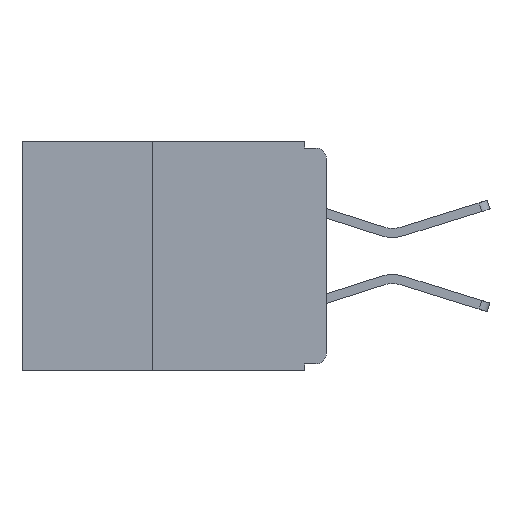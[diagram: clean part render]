
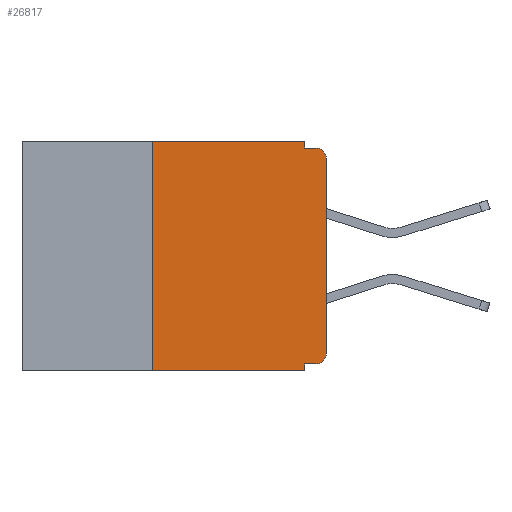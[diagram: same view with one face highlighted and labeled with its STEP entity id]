
A CAD part, left-side view. The second image highlights one B-rep face of the part: STEP entity #26817.
In plain terms, the highlighted planar face has unit normal (-1, 0, 0).
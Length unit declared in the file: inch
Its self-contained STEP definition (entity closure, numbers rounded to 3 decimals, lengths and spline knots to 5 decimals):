
#557 = DIRECTION ( 'NONE',  ( 0., 0., -1. ) ) ;
#1040 = CARTESIAN_POINT ( 'NONE',  ( 0., 0.25, -0.33 ) ) ;
#1101 = ORIENTED_EDGE ( 'NONE', *, *, #28838, .T. ) ;
#1144 = VECTOR ( 'NONE', #1265, 39.37008 ) ;
#1265 = DIRECTION ( 'NONE',  ( 0., -1., 0. ) ) ;
#1448 = CARTESIAN_POINT ( 'NONE',  ( 0., 0.437, 0. ) ) ;
#2435 = AXIS2_PLACEMENT_3D ( 'NONE', #10925, #27339, #13298 ) ;
#3317 = CARTESIAN_POINT ( 'NONE',  ( 0., 0.031, -0.33 ) ) ;
#3629 = AXIS2_PLACEMENT_3D ( 'NONE', #13656, #29959, #16044 ) ;
#4283 = FACE_OUTER_BOUND ( 'NONE', #9705, .T. ) ;
#4309 = CIRCLE ( 'NONE', #2435, 0.015 ) ;
#4609 = LINE ( 'NONE', #1040, #6136 ) ;
#4827 = CARTESIAN_POINT ( 'NONE',  ( 0., 0.437, -0.33 ) ) ;
#5340 = ORIENTED_EDGE ( 'NONE', *, *, #13169, .F. ) ;
#5691 = ORIENTED_EDGE ( 'NONE', *, *, #6755, .T. ) ;
#5757 = DIRECTION ( 'NONE',  ( 0., 0., -1. ) ) ;
#5878 = VERTEX_POINT ( 'NONE', #7886 ) ;
#5904 = DIRECTION ( 'NONE',  ( 0., 0., 1. ) ) ;
#6136 = VECTOR ( 'NONE', #5904, 39.37008 ) ;
#6251 = VECTOR ( 'NONE', #20528, 39.37008 ) ;
#6602 = VECTOR ( 'NONE', #28441, 39.37008 ) ;
#6671 = VERTEX_POINT ( 'NONE', #20366 ) ;
#6755 = EDGE_CURVE ( 'NONE', #5878, #24938, #7112, .T. ) ;
#7112 = CIRCLE ( 'NONE', #3629, 0.015 ) ;
#7171 = CARTESIAN_POINT ( 'NONE',  ( 0., 0.031, -0.33 ) ) ;
#7465 = CARTESIAN_POINT ( 'NONE',  ( 0., 0.25, -0.33 ) ) ;
#7669 = CARTESIAN_POINT ( 'NONE',  ( 0., 0., -0.305 ) ) ;
#7886 = CARTESIAN_POINT ( 'NONE',  ( 0., 0.015, -0.32 ) ) ;
#7937 = VECTOR ( 'NONE', #30121, 39.37008 ) ;
#8314 = CARTESIAN_POINT ( 'NONE',  ( 0., 0., -0.025 ) ) ;
#8569 = CARTESIAN_POINT ( 'NONE',  ( 0., 0., -0.01 ) ) ;
#9251 = ORIENTED_EDGE ( 'NONE', *, *, #11763, .F. ) ;
#9355 = LINE ( 'NONE', #3317, #21174 ) ;
#9705 = EDGE_LOOP ( 'NONE', ( #1101, #9840, #13151, #24404, #18712, #21427, #24216, #9251, #5340, #5691 ) ) ;
#9840 = ORIENTED_EDGE ( 'NONE', *, *, #9993, .T. ) ;
#9993 = EDGE_CURVE ( 'NONE', #22914, #6671, #4309, .T. ) ;
#10048 = CARTESIAN_POINT ( 'NONE',  ( 0., 0.031, -0.32 ) ) ;
#10231 = VECTOR ( 'NONE', #23945, 39.37008 ) ;
#10925 = CARTESIAN_POINT ( 'NONE',  ( 0., 0.015, -0.025 ) ) ;
#10972 = LINE ( 'NONE', #19273, #10231 ) ;
#11763 = EDGE_CURVE ( 'NONE', #19032, #14661, #9355, .T. ) ;
#12555 = PLANE ( 'NONE',  #16244 ) ;
#12974 = LINE ( 'NONE', #4827, #6602 ) ;
#13127 = EDGE_CURVE ( 'NONE', #30476, #18614, #13366, .T. ) ;
#13151 = ORIENTED_EDGE ( 'NONE', *, *, #21045, .F. ) ;
#13169 = EDGE_CURVE ( 'NONE', #5878, #19032, #24374, .T. ) ;
#13284 = CARTESIAN_POINT ( 'NONE',  ( 0., 0.031, 0. ) ) ;
#13298 = DIRECTION ( 'NONE',  ( 0., 0., -1. ) ) ;
#13358 = EDGE_CURVE ( 'NONE', #13422, #14661, #12974, .T. ) ;
#13366 = LINE ( 'NONE', #1448, #6251 ) ;
#13422 = VERTEX_POINT ( 'NONE', #7465 ) ;
#13656 = CARTESIAN_POINT ( 'NONE',  ( 0., 0.015, -0.305 ) ) ;
#13910 = LINE ( 'NONE', #8569, #1144 ) ;
#14661 = VERTEX_POINT ( 'NONE', #7171 ) ;
#14945 = DIRECTION ( 'NONE',  ( 1., 0., 0. ) ) ;
#14947 = EDGE_CURVE ( 'NONE', #13422, #30476, #4609, .T. ) ;
#16002 = CARTESIAN_POINT ( 'NONE',  ( 0., 0., -0.32 ) ) ;
#16044 = DIRECTION ( 'NONE',  ( 0., 0., -1. ) ) ;
#16244 = AXIS2_PLACEMENT_3D ( 'NONE', #28908, #14945, #557 ) ;
#16524 = EDGE_CURVE ( 'NONE', #18614, #22450, #10972, .T. ) ;
#17443 = VECTOR ( 'NONE', #18385, 39.37008 ) ;
#18385 = DIRECTION ( 'NONE',  ( 0., 1., 0. ) ) ;
#18614 = VERTEX_POINT ( 'NONE', #13284 ) ;
#18712 = ORIENTED_EDGE ( 'NONE', *, *, #13127, .F. ) ;
#19032 = VERTEX_POINT ( 'NONE', #10048 ) ;
#19273 = CARTESIAN_POINT ( 'NONE',  ( 0., 0.031, 0. ) ) ;
#20366 = CARTESIAN_POINT ( 'NONE',  ( 0., 0.015, -0.01 ) ) ;
#20528 = DIRECTION ( 'NONE',  ( 0., -1., 0. ) ) ;
#21045 = EDGE_CURVE ( 'NONE', #22450, #6671, #13910, .T. ) ;
#21174 = VECTOR ( 'NONE', #5757, 39.37008 ) ;
#21242 = LINE ( 'NONE', #27857, #7937 ) ;
#21427 = ORIENTED_EDGE ( 'NONE', *, *, #14947, .F. ) ;
#22450 = VERTEX_POINT ( 'NONE', #25422 ) ;
#22914 = VERTEX_POINT ( 'NONE', #8314 ) ;
#23945 = DIRECTION ( 'NONE',  ( 0., 0., -1. ) ) ;
#24216 = ORIENTED_EDGE ( 'NONE', *, *, #13358, .T. ) ;
#24374 = LINE ( 'NONE', #16002, #17443 ) ;
#24404 = ORIENTED_EDGE ( 'NONE', *, *, #16524, .F. ) ;
#24938 = VERTEX_POINT ( 'NONE', #7669 ) ;
#25422 = CARTESIAN_POINT ( 'NONE',  ( 0., 0.031, -0.01 ) ) ;
#26817 = ADVANCED_FACE ( 'NONE', ( #4283 ), #12555, .F. ) ;
#27339 = DIRECTION ( 'NONE',  ( -1., 0., 0. ) ) ;
#27857 = CARTESIAN_POINT ( 'NONE',  ( 0., 0., 0. ) ) ;
#28441 = DIRECTION ( 'NONE',  ( 0., -1., 0. ) ) ;
#28838 = EDGE_CURVE ( 'NONE', #24938, #22914, #21242, .T. ) ;
#28908 = CARTESIAN_POINT ( 'NONE',  ( 0., 0.437, 0. ) ) ;
#29337 = CARTESIAN_POINT ( 'NONE',  ( 0., 0.25, 0. ) ) ;
#29959 = DIRECTION ( 'NONE',  ( -1., 0., 0. ) ) ;
#30121 = DIRECTION ( 'NONE',  ( 0., 0., 1. ) ) ;
#30476 = VERTEX_POINT ( 'NONE', #29337 ) ;
